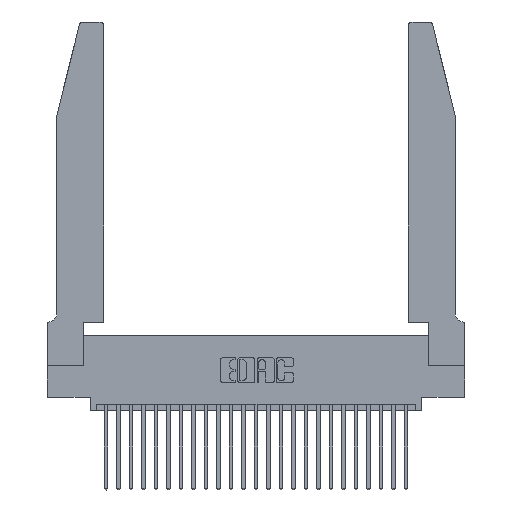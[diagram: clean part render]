
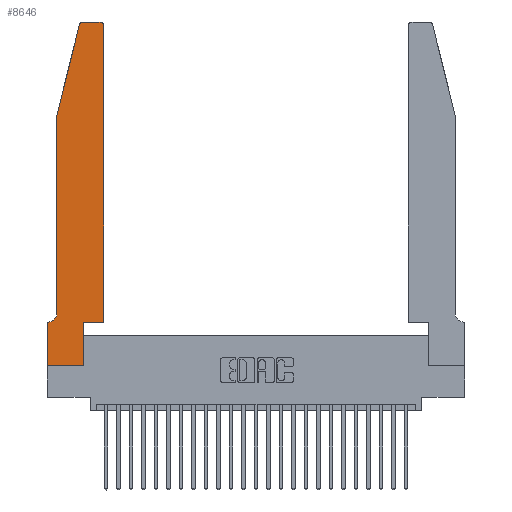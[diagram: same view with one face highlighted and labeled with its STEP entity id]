
A CAD part, top view. The second image highlights one B-rep face of the part: STEP entity #8646.
In plain terms, the highlighted planar face has unit normal (0, 0, 1).
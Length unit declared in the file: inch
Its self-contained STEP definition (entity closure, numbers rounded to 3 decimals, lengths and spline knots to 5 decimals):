
#460 = ORIENTED_EDGE ( 'NONE', *, *, #13783, .T. ) ;
#759 = DIRECTION ( 'NONE',  ( 1., 0., 0. ) ) ;
#935 = AXIS2_PLACEMENT_3D ( 'NONE', #21731, #13533, #1116 ) ;
#1116 = DIRECTION ( 'NONE',  ( 1., 0., 0. ) ) ;
#1893 = DIRECTION ( 'NONE',  ( 1., 0., 0. ) ) ;
#2276 = CARTESIAN_POINT ( 'NONE',  ( 0., 0., 0.37 ) ) ;
#2605 = DIRECTION ( 'NONE',  ( -1., 0., 0. ) ) ;
#2675 = CARTESIAN_POINT ( 'NONE',  ( 0.4505, 0.35, 0.37 ) ) ;
#3339 = CARTESIAN_POINT ( 'NONE',  ( 0.2865, 0.35, 0.37 ) ) ;
#4019 = EDGE_CURVE ( 'NONE', #10103, #19026, #10868, .T. ) ;
#5429 = CARTESIAN_POINT ( 'NONE',  ( 0.284, 2.75, 0.37 ) ) ;
#5611 = ORIENTED_EDGE ( 'NONE', *, *, #12498, .T. ) ;
#5828 = EDGE_LOOP ( 'NONE', ( #15679, #17596, #460, #11463, #6294, #21981, #7140, #22171, #5611, #14924, #10543, #22165 ) ) ;
#6126 = CARTESIAN_POINT ( 'NONE',  ( 0.2865, 0., 0.37 ) ) ;
#6294 = ORIENTED_EDGE ( 'NONE', *, *, #11741, .T. ) ;
#6520 = VERTEX_POINT ( 'NONE', #6126 ) ;
#6930 = DIRECTION ( 'NONE',  ( -0.239, -0.971, 0. ) ) ;
#7018 = VECTOR ( 'NONE', #13943, 39.37008 ) ;
#7140 = ORIENTED_EDGE ( 'NONE', *, *, #18227, .T. ) ;
#7452 = CARTESIAN_POINT ( 'NONE',  ( 0.2605, 2.75, 0.37 ) ) ;
#7602 = VECTOR ( 'NONE', #6930, 39.37008 ) ;
#7638 = VERTEX_POINT ( 'NONE', #11419 ) ;
#7842 = VECTOR ( 'NONE', #11496, 39.37008 ) ;
#7931 = CARTESIAN_POINT ( 'NONE',  ( 0.25487, 2.72718, 0.37 ) ) ;
#8354 = CARTESIAN_POINT ( 'NONE',  ( 0.0055, 0.42, 0.37 ) ) ;
#8527 = DIRECTION ( 'NONE',  ( 0., -1., 0. ) ) ;
#8646 = ADVANCED_FACE ( 'NONE', ( #10928 ), #11914, .T. ) ;
#8761 = DIRECTION ( 'NONE',  ( 1., 0., 0. ) ) ;
#8977 = EDGE_CURVE ( 'NONE', #19026, #18406, #18054, .T. ) ;
#9065 = CARTESIAN_POINT ( 'NONE',  ( 0.4505, 2.72, 0.37 ) ) ;
#9281 = LINE ( 'NONE', #21129, #21570 ) ;
#9342 = VERTEX_POINT ( 'NONE', #20608 ) ;
#9419 = EDGE_CURVE ( 'NONE', #25905, #21826, #23605, .T. ) ;
#9561 = EDGE_CURVE ( 'NONE', #9342, #25905, #9762, .T. ) ;
#9762 = LINE ( 'NONE', #7452, #7842 ) ;
#10103 = VERTEX_POINT ( 'NONE', #3339 ) ;
#10543 = ORIENTED_EDGE ( 'NONE', *, *, #8977, .T. ) ;
#10582 = AXIS2_PLACEMENT_3D ( 'NONE', #13835, #15910, #26382 ) ;
#10817 = VERTEX_POINT ( 'NONE', #11568 ) ;
#10868 = LINE ( 'NONE', #12390, #13795 ) ;
#10928 = FACE_OUTER_BOUND ( 'NONE', #5828, .T. ) ;
#11419 = CARTESIAN_POINT ( 'NONE',  ( 0., 0., 0.37 ) ) ;
#11463 = ORIENTED_EDGE ( 'NONE', *, *, #13659, .T. ) ;
#11496 = DIRECTION ( 'NONE',  ( -1., 0., 0. ) ) ;
#11568 = CARTESIAN_POINT ( 'NONE',  ( 0.0055, 0.35, 0.37 ) ) ;
#11741 = EDGE_CURVE ( 'NONE', #11786, #10817, #23545, .T. ) ;
#11786 = VERTEX_POINT ( 'NONE', #26754 ) ;
#11914 = PLANE ( 'NONE',  #10582 ) ;
#12390 = CARTESIAN_POINT ( 'NONE',  ( 0.4505, 0.35, 0.37 ) ) ;
#12498 = EDGE_CURVE ( 'NONE', #6520, #10103, #21557, .T. ) ;
#12843 = CARTESIAN_POINT ( 'NONE',  ( 0.0755, 0.35, 0.37 ) ) ;
#13157 = CARTESIAN_POINT ( 'NONE',  ( 0.0755, 2., 0.37 ) ) ;
#13165 = CARTESIAN_POINT ( 'NONE',  ( 0.284, 2.72, 0.37 ) ) ;
#13401 = LINE ( 'NONE', #13157, #7602 ) ;
#13533 = DIRECTION ( 'NONE',  ( 0., 0., 1. ) ) ;
#13659 = EDGE_CURVE ( 'NONE', #21444, #11786, #25701, .T. ) ;
#13678 = DIRECTION ( 'NONE',  ( 0., -1., 0. ) ) ;
#13783 = EDGE_CURVE ( 'NONE', #21826, #21444, #13401, .T. ) ;
#13795 = VECTOR ( 'NONE', #1893, 39.37008 ) ;
#13835 = CARTESIAN_POINT ( 'NONE',  ( 0., 0.35, 0.37 ) ) ;
#13943 = DIRECTION ( 'NONE',  ( 0., 1., 0. ) ) ;
#13960 = LINE ( 'NONE', #12843, #15592 ) ;
#14005 = CIRCLE ( 'NONE', #935, 0.03 ) ;
#14624 = EDGE_CURVE ( 'NONE', #18406, #9342, #14005, .T. ) ;
#14679 = DIRECTION ( 'NONE',  ( -1., 0., 0. ) ) ;
#14924 = ORIENTED_EDGE ( 'NONE', *, *, #4019, .T. ) ;
#15103 = AXIS2_PLACEMENT_3D ( 'NONE', #13165, #15177, #759 ) ;
#15177 = DIRECTION ( 'NONE',  ( 0., 0., 1. ) ) ;
#15401 = CARTESIAN_POINT ( 'NONE',  ( 0.0755, 2., 0.37 ) ) ;
#15573 = EDGE_CURVE ( 'NONE', #10817, #21809, #13960, .T. ) ;
#15592 = VECTOR ( 'NONE', #2605, 39.37008 ) ;
#15679 = ORIENTED_EDGE ( 'NONE', *, *, #9561, .T. ) ;
#15898 = DIRECTION ( 'NONE',  ( 0., 1., 0. ) ) ;
#15910 = DIRECTION ( 'NONE',  ( 0., 0., 1. ) ) ;
#16666 = VECTOR ( 'NONE', #8527, 39.37008 ) ;
#17066 = EDGE_CURVE ( 'NONE', #7638, #6520, #9281, .T. ) ;
#17288 = VECTOR ( 'NONE', #13678, 39.37008 ) ;
#17394 = VECTOR ( 'NONE', #15898, 39.37008 ) ;
#17596 = ORIENTED_EDGE ( 'NONE', *, *, #9419, .T. ) ;
#18054 = LINE ( 'NONE', #2675, #17394 ) ;
#18227 = EDGE_CURVE ( 'NONE', #21809, #7638, #25729, .T. ) ;
#18406 = VERTEX_POINT ( 'NONE', #9065 ) ;
#19026 = VERTEX_POINT ( 'NONE', #26476 ) ;
#20382 = CARTESIAN_POINT ( 'NONE',  ( 0., 0.35, 0.37 ) ) ;
#20608 = CARTESIAN_POINT ( 'NONE',  ( 0.4205, 2.75, 0.37 ) ) ;
#21129 = CARTESIAN_POINT ( 'NONE',  ( 0., 0., 0.37 ) ) ;
#21444 = VERTEX_POINT ( 'NONE', #25374 ) ;
#21557 = LINE ( 'NONE', #22064, #7018 ) ;
#21570 = VECTOR ( 'NONE', #8761, 39.37008 ) ;
#21731 = CARTESIAN_POINT ( 'NONE',  ( 0.4205, 2.72, 0.37 ) ) ;
#21809 = VERTEX_POINT ( 'NONE', #20382 ) ;
#21826 = VERTEX_POINT ( 'NONE', #7931 ) ;
#21981 = ORIENTED_EDGE ( 'NONE', *, *, #15573, .T. ) ;
#22064 = CARTESIAN_POINT ( 'NONE',  ( 0.2865, 0.35, 0.37 ) ) ;
#22165 = ORIENTED_EDGE ( 'NONE', *, *, #14624, .T. ) ;
#22171 = ORIENTED_EDGE ( 'NONE', *, *, #17066, .T. ) ;
#22885 = DIRECTION ( 'NONE',  ( 0., 0., -1. ) ) ;
#23545 = CIRCLE ( 'NONE', #24473, 0.07 ) ;
#23605 = CIRCLE ( 'NONE', #15103, 0.03 ) ;
#24473 = AXIS2_PLACEMENT_3D ( 'NONE', #8354, #22885, #14679 ) ;
#25374 = CARTESIAN_POINT ( 'NONE',  ( 0.0755, 2., 0.37 ) ) ;
#25701 = LINE ( 'NONE', #15401, #17288 ) ;
#25729 = LINE ( 'NONE', #2276, #16666 ) ;
#25905 = VERTEX_POINT ( 'NONE', #5429 ) ;
#26382 = DIRECTION ( 'NONE',  ( 1., 0., 0. ) ) ;
#26476 = CARTESIAN_POINT ( 'NONE',  ( 0.4505, 0.35, 0.37 ) ) ;
#26754 = CARTESIAN_POINT ( 'NONE',  ( 0.0755, 0.42, 0.37 ) ) ;
